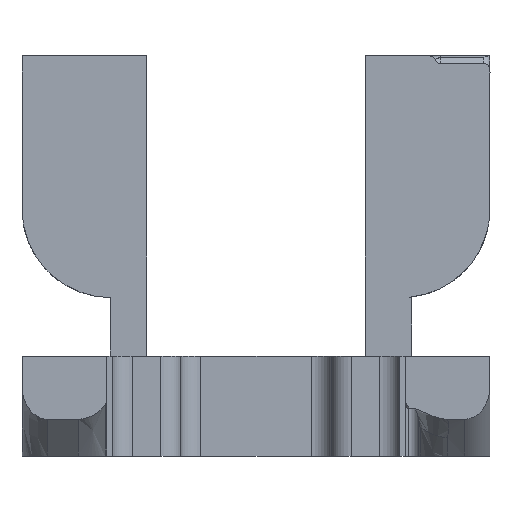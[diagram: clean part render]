
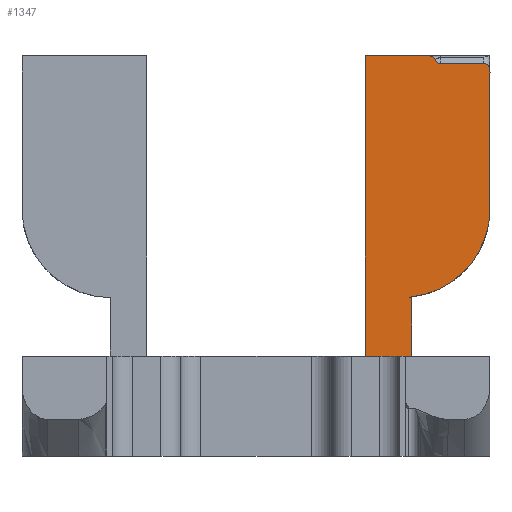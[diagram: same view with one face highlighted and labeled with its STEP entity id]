
A CAD part, front view. The second image highlights one B-rep face of the part: STEP entity #1347.
In plain terms, the highlighted planar face has unit normal (0, -1, 0).
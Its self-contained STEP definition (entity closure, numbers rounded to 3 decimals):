
#2 = CARTESIAN_POINT ( 'NONE',  ( 30.782, 36.168, 237.745 ) ) ;
#32 = LINE ( 'NONE', #2426, #3263 ) ;
#33 = CARTESIAN_POINT ( 'NONE',  ( 31.282, 36.168, 237.037 ) ) ;
#36 = VERTEX_POINT ( 'NONE', #1060 ) ;
#41 = CARTESIAN_POINT ( 'NONE',  ( 26.644, 36.168, 238.327 ) ) ;
#64 = DIRECTION ( 'NONE',  ( 0., 0., 1. ) ) ;
#72 = CARTESIAN_POINT ( 'NONE',  ( 27.03, 36.168, 237.849 ) ) ;
#182 = CARTESIAN_POINT ( 'NONE',  ( 31.282, 36.168, 226.207 ) ) ;
#207 = B_SPLINE_CURVE_WITH_KNOTS ( 'NONE', 3,
 ( #3634, #41, #3142, #3464 ),
 .UNSPECIFIED., .F., .F.,
 ( 4, 4 ),
 ( 0., 0.001 ),
 .UNSPECIFIED. ) ;
#259 = VECTOR ( 'NONE', #3280, 1000. ) ;
#277 = CARTESIAN_POINT ( 'NONE',  ( 24.225, 36.168, 226.207 ) ) ;
#313 = CARTESIAN_POINT ( 'NONE',  ( 31.075, 36.168, 237.745 ) ) ;
#547 = DIRECTION ( 'NONE',  ( 0., -1., 0. ) ) ;
#549 = VECTOR ( 'NONE', #2170, 1000. ) ;
#567 = ORIENTED_EDGE ( 'NONE', *, *, #903, .F. ) ;
#593 = DIRECTION ( 'NONE',  ( 1., 0., 0. ) ) ;
#606 = LINE ( 'NONE', #1051, #2151 ) ;
#625 = EDGE_CURVE ( 'NONE', #4024, #2401, #1006, .T. ) ;
#631 = CARTESIAN_POINT ( 'NONE',  ( 31.282, 36.168, 237.452 ) ) ;
#653 =( BOUNDED_CURVE ( )  B_SPLINE_CURVE ( 3, ( #3158, #1600, #72, #2239 ),
 .UNSPECIFIED., .F., .F. ) 
 B_SPLINE_CURVE_WITH_KNOTS ( ( 4, 4 ),
 ( 0., 0.941 ),
 .UNSPECIFIED. ) 
 CURVE ( )  GEOMETRIC_REPRESENTATION_ITEM ( )  RATIONAL_B_SPLINE_CURVE ( ( 1., 0.928, 0.928, 1. ) ) 
 REPRESENTATION_ITEM ( '' )  );
#825 = CARTESIAN_POINT ( 'NONE',  ( 26.934, 36.168, 238.035 ) ) ;
#892 = DIRECTION ( 'NONE',  ( -1., 0., 0. ) ) ;
#893 = CARTESIAN_POINT ( 'NONE',  ( 26.442, 36.168, 238.327 ) ) ;
#900 = CARTESIAN_POINT ( 'NONE',  ( 31.282, 36.168, 226.207 ) ) ;
#903 = EDGE_CURVE ( 'NONE', #1415, #2834, #207, .T. ) ;
#949 = EDGE_CURVE ( 'NONE', #2365, #2834, #653, .T. ) ;
#1006 = LINE ( 'NONE', #1909, #4018 ) ;
#1051 = CARTESIAN_POINT ( 'NONE',  ( 21.4, 36.168, 206.577 ) ) ;
#1060 = CARTESIAN_POINT ( 'NONE',  ( 21.4, 36.168, 214.515 ) ) ;
#1222 = CARTESIAN_POINT ( 'NONE',  ( 30.782, 36.168, 237.745 ) ) ;
#1347 = ADVANCED_FACE ( 'NONE', ( #2470 ), #2406, .T. ) ;
#1371 = LINE ( 'NONE', #3426, #549 ) ;
#1415 = VERTEX_POINT ( 'NONE', #893 ) ;
#1486 =( BOUNDED_CURVE ( )  B_SPLINE_CURVE ( 3, ( #2, #313, #631, #2794 ),
 .UNSPECIFIED., .F., .T. ) 
 B_SPLINE_CURVE_WITH_KNOTS ( ( 4, 4 ),
 ( 3.142, 4.712 ),
 .UNSPECIFIED. ) 
 CURVE ( )  GEOMETRIC_REPRESENTATION_ITEM ( )  RATIONAL_B_SPLINE_CURVE ( ( 1., 0.805, 0.805, 1. ) ) 
 REPRESENTATION_ITEM ( '' )  );
#1502 = ORIENTED_EDGE ( 'NONE', *, *, #2504, .T. ) ;
#1534 = ORIENTED_EDGE ( 'NONE', *, *, #3709, .F. ) ;
#1586 = CARTESIAN_POINT ( 'NONE',  ( 27.338, 36.168, 237.745 ) ) ;
#1600 = CARTESIAN_POINT ( 'NONE',  ( 27.175, 36.168, 237.745 ) ) ;
#1636 = VERTEX_POINT ( 'NONE', #1853 ) ;
#1696 = AXIS2_PLACEMENT_3D ( 'NONE', #277, #2446, #593 ) ;
#1796 = VERTEX_POINT ( 'NONE', #900 ) ;
#1839 = ORIENTED_EDGE ( 'NONE', *, *, #625, .T. ) ;
#1853 = CARTESIAN_POINT ( 'NONE',  ( 21.4, 36.168, 238.327 ) ) ;
#1909 = CARTESIAN_POINT ( 'NONE',  ( 25.077, 36.168, 231.964 ) ) ;
#2136 = DIRECTION ( 'NONE',  ( 1., 0., 0. ) ) ;
#2151 = VECTOR ( 'NONE', #3218, 1000. ) ;
#2170 = DIRECTION ( 'NONE',  ( 1., 0., 0. ) ) ;
#2239 = CARTESIAN_POINT ( 'NONE',  ( 26.934, 36.168, 238.035 ) ) ;
#2365 = VERTEX_POINT ( 'NONE', #1586 ) ;
#2401 = VERTEX_POINT ( 'NONE', #3143 ) ;
#2406 = PLANE ( 'NONE',  #3286 ) ;
#2424 = ORIENTED_EDGE ( 'NONE', *, *, #2780, .T. ) ;
#2426 = CARTESIAN_POINT ( 'NONE',  ( 12.715, 36.168, 237.745 ) ) ;
#2446 = DIRECTION ( 'NONE',  ( 0., 1., 0. ) ) ;
#2470 = FACE_OUTER_BOUND ( 'NONE', #2790, .T. ) ;
#2504 = EDGE_CURVE ( 'NONE', #1636, #36, #606, .T. ) ;
#2716 = DIRECTION ( 'NONE',  ( 1., 0., 0. ) ) ;
#2718 = ORIENTED_EDGE ( 'NONE', *, *, #3641, .T. ) ;
#2756 = CARTESIAN_POINT ( 'NONE',  ( 27.003, 36.168, 238.327 ) ) ;
#2780 = EDGE_CURVE ( 'NONE', #1796, #3874, #3376, .T. ) ;
#2790 = EDGE_LOOP ( 'NONE', ( #1839, #1534, #2424, #3192, #2718, #3287, #567, #3047, #1502, #3796 ) ) ;
#2794 = CARTESIAN_POINT ( 'NONE',  ( 31.282, 36.168, 237.037 ) ) ;
#2834 = VERTEX_POINT ( 'NONE', #825 ) ;
#3038 = VERTEX_POINT ( 'NONE', #1222 ) ;
#3047 = ORIENTED_EDGE ( 'NONE', *, *, #3727, .F. ) ;
#3049 = VECTOR ( 'NONE', #2136, 1000. ) ;
#3103 = EDGE_CURVE ( 'NONE', #3038, #3874, #1486, .T. ) ;
#3126 = EDGE_CURVE ( 'NONE', #36, #4024, #1371, .T. ) ;
#3132 = CIRCLE ( 'NONE', #1696, 7.057 ) ;
#3142 = CARTESIAN_POINT ( 'NONE',  ( 26.841, 36.168, 238.216 ) ) ;
#3143 = CARTESIAN_POINT ( 'NONE',  ( 25.077, 36.168, 219.202 ) ) ;
#3158 = CARTESIAN_POINT ( 'NONE',  ( 27.338, 36.168, 237.745 ) ) ;
#3192 = ORIENTED_EDGE ( 'NONE', *, *, #3103, .F. ) ;
#3218 = DIRECTION ( 'NONE',  ( 0., 0., -1. ) ) ;
#3263 = VECTOR ( 'NONE', #892, 1000. ) ;
#3280 = DIRECTION ( 'NONE',  ( 0., 0., 1. ) ) ;
#3286 = AXIS2_PLACEMENT_3D ( 'NONE', #3650, #547, #2716 ) ;
#3287 = ORIENTED_EDGE ( 'NONE', *, *, #949, .T. ) ;
#3376 = LINE ( 'NONE', #182, #259 ) ;
#3426 = CARTESIAN_POINT ( 'NONE',  ( -6.693, 36.168, 214.515 ) ) ;
#3464 = CARTESIAN_POINT ( 'NONE',  ( 26.934, 36.168, 238.035 ) ) ;
#3634 = CARTESIAN_POINT ( 'NONE',  ( 26.442, 36.168, 238.327 ) ) ;
#3641 = EDGE_CURVE ( 'NONE', #3038, #2365, #32, .T. ) ;
#3650 = CARTESIAN_POINT ( 'NONE',  ( -6.693, 36.168, 0. ) ) ;
#3709 = EDGE_CURVE ( 'NONE', #1796, #2401, #3132, .T. ) ;
#3727 = EDGE_CURVE ( 'NONE', #1636, #1415, #3987, .T. ) ;
#3796 = ORIENTED_EDGE ( 'NONE', *, *, #3126, .T. ) ;
#3843 = CARTESIAN_POINT ( 'NONE',  ( 25.077, 36.168, 214.515 ) ) ;
#3874 = VERTEX_POINT ( 'NONE', #33 ) ;
#3987 = LINE ( 'NONE', #2756, #3049 ) ;
#4018 = VECTOR ( 'NONE', #64, 1000. ) ;
#4024 = VERTEX_POINT ( 'NONE', #3843 ) ;
